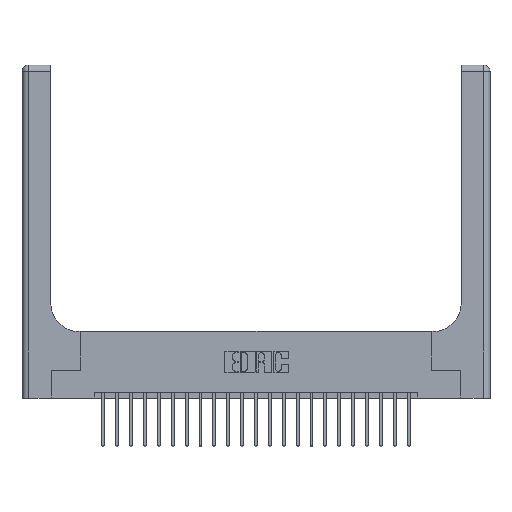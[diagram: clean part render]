
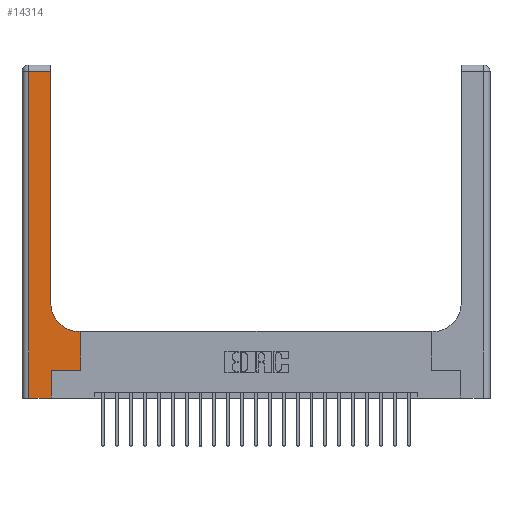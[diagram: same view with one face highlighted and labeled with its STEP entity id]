
A CAD part, top view. The second image highlights one B-rep face of the part: STEP entity #14314.
In plain terms, the highlighted planar face has unit normal (0, 0, 1).
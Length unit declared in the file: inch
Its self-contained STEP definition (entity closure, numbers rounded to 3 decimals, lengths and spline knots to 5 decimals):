
#90 = CARTESIAN_POINT ( 'NONE',  ( 0.528, 0.25, 0.37 ) ) ;
#237 = CARTESIAN_POINT ( 'NONE',  ( 0.26, 0.85, 0.37 ) ) ;
#521 = LINE ( 'NONE', #18721, #15251 ) ;
#637 = FACE_OUTER_BOUND ( 'NONE', #8302, .T. ) ;
#1645 = VECTOR ( 'NONE', #20499, 39.37008 ) ;
#1762 = ORIENTED_EDGE ( 'NONE', *, *, #19918, .T. ) ;
#1767 = CARTESIAN_POINT ( 'NONE',  ( 0.528, 0.25, 0.37 ) ) ;
#1967 = ORIENTED_EDGE ( 'NONE', *, *, #8684, .T. ) ;
#2115 = AXIS2_PLACEMENT_3D ( 'NONE', #13192, #11765, #16937 ) ;
#2362 = CARTESIAN_POINT ( 'NONE',  ( 0., 2.94, 0.37 ) ) ;
#2823 = EDGE_CURVE ( 'NONE', #16064, #22870, #18505, .T. ) ;
#2943 = CARTESIAN_POINT ( 'NONE',  ( 0.265, 0., 0.37 ) ) ;
#3073 = DIRECTION ( 'NONE',  ( 1., 0., 0. ) ) ;
#3190 = CARTESIAN_POINT ( 'NONE',  ( 0.51, 0.85, 0.37 ) ) ;
#4255 = VECTOR ( 'NONE', #6869, 39.37008 ) ;
#4776 = DIRECTION ( 'NONE',  ( -1., 0., 0. ) ) ;
#4929 = EDGE_CURVE ( 'NONE', #17210, #16064, #18693, .T. ) ;
#5372 = EDGE_CURVE ( 'NONE', #14611, #19158, #14999, .T. ) ;
#5555 = ORIENTED_EDGE ( 'NONE', *, *, #4929, .T. ) ;
#5821 = CARTESIAN_POINT ( 'NONE',  ( 0.06, 3., 0.37 ) ) ;
#6184 = LINE ( 'NONE', #22422, #21962 ) ;
#6869 = DIRECTION ( 'NONE',  ( 1., 0., 0. ) ) ;
#6930 = VECTOR ( 'NONE', #11194, 39.37008 ) ;
#7062 = CARTESIAN_POINT ( 'NONE',  ( 0.265, 0.25, 0.37 ) ) ;
#7565 = DIRECTION ( 'NONE',  ( 0., 1., 0. ) ) ;
#7574 = ORIENTED_EDGE ( 'NONE', *, *, #20050, .T. ) ;
#7586 = VECTOR ( 'NONE', #9031, 39.37008 ) ;
#8020 = LINE ( 'NONE', #8369, #1645 ) ;
#8302 = EDGE_LOOP ( 'NONE', ( #16975, #5555, #13541, #1967, #1762, #12781, #22133, #13637, #7574 ) ) ;
#8369 = CARTESIAN_POINT ( 'NONE',  ( 0.265, 0., 0.37 ) ) ;
#8684 = EDGE_CURVE ( 'NONE', #22870, #22926, #17682, .T. ) ;
#8923 = DIRECTION ( 'NONE',  ( 0., 1., 0. ) ) ;
#9031 = DIRECTION ( 'NONE',  ( 1., 0., 0. ) ) ;
#10506 = CARTESIAN_POINT ( 'NONE',  ( 0.26, 2.94, 0.37 ) ) ;
#10559 = LINE ( 'NONE', #1767, #21582 ) ;
#11194 = DIRECTION ( 'NONE',  ( -1., 0., 0. ) ) ;
#11668 = CARTESIAN_POINT ( 'NONE',  ( 0.51, 0.6, 0.37 ) ) ;
#11765 = DIRECTION ( 'NONE',  ( 0., 0., -1. ) ) ;
#12781 = ORIENTED_EDGE ( 'NONE', *, *, #5372, .T. ) ;
#13124 = DIRECTION ( 'NONE',  ( 0., -1., 0. ) ) ;
#13192 = CARTESIAN_POINT ( 'NONE',  ( 0., 3., 0.37 ) ) ;
#13259 = EDGE_CURVE ( 'NONE', #19158, #13663, #10559, .T. ) ;
#13368 = EDGE_CURVE ( 'NONE', #13663, #18626, #6184, .T. ) ;
#13541 = ORIENTED_EDGE ( 'NONE', *, *, #2823, .T. ) ;
#13637 = ORIENTED_EDGE ( 'NONE', *, *, #13368, .T. ) ;
#13663 = VERTEX_POINT ( 'NONE', #16270 ) ;
#14314 = ADVANCED_FACE ( 'NONE', ( #637 ), #22479, .F. ) ;
#14323 = CARTESIAN_POINT ( 'NONE',  ( 0.265, 0.25, 0.37 ) ) ;
#14611 = VERTEX_POINT ( 'NONE', #7062 ) ;
#14999 = LINE ( 'NONE', #14323, #7586 ) ;
#15178 = AXIS2_PLACEMENT_3D ( 'NONE', #3190, #22949, #3073 ) ;
#15251 = VECTOR ( 'NONE', #7565, 39.37008 ) ;
#16064 = VERTEX_POINT ( 'NONE', #21519 ) ;
#16270 = CARTESIAN_POINT ( 'NONE',  ( 0.528, 0.6, 0.37 ) ) ;
#16490 = VERTEX_POINT ( 'NONE', #237 ) ;
#16937 = DIRECTION ( 'NONE',  ( -1., 0., 0. ) ) ;
#16975 = ORIENTED_EDGE ( 'NONE', *, *, #22258, .T. ) ;
#17210 = VERTEX_POINT ( 'NONE', #10506 ) ;
#17227 = CARTESIAN_POINT ( 'NONE',  ( 0., 0., 0.37 ) ) ;
#17682 = LINE ( 'NONE', #17227, #4255 ) ;
#18483 = VECTOR ( 'NONE', #13124, 39.37008 ) ;
#18505 = LINE ( 'NONE', #5821, #18483 ) ;
#18626 = VERTEX_POINT ( 'NONE', #11668 ) ;
#18690 = CARTESIAN_POINT ( 'NONE',  ( 0.06, 0., 0.37 ) ) ;
#18693 = LINE ( 'NONE', #2362, #6930 ) ;
#18721 = CARTESIAN_POINT ( 'NONE',  ( 0.26, 3., 0.37 ) ) ;
#19158 = VERTEX_POINT ( 'NONE', #90 ) ;
#19918 = EDGE_CURVE ( 'NONE', #22926, #14611, #8020, .T. ) ;
#20050 = EDGE_CURVE ( 'NONE', #18626, #16490, #22674, .T. ) ;
#20499 = DIRECTION ( 'NONE',  ( 0., 1., 0. ) ) ;
#21519 = CARTESIAN_POINT ( 'NONE',  ( 0.06, 2.94, 0.37 ) ) ;
#21582 = VECTOR ( 'NONE', #8923, 39.37008 ) ;
#21962 = VECTOR ( 'NONE', #4776, 39.37008 ) ;
#22133 = ORIENTED_EDGE ( 'NONE', *, *, #13259, .T. ) ;
#22258 = EDGE_CURVE ( 'NONE', #16490, #17210, #521, .T. ) ;
#22422 = CARTESIAN_POINT ( 'NONE',  ( 0.26, 0.6, 0.37 ) ) ;
#22479 = PLANE ( 'NONE',  #2115 ) ;
#22674 = CIRCLE ( 'NONE', #15178, 0.25 ) ;
#22870 = VERTEX_POINT ( 'NONE', #18690 ) ;
#22926 = VERTEX_POINT ( 'NONE', #2943 ) ;
#22949 = DIRECTION ( 'NONE',  ( 0., 0., -1. ) ) ;
